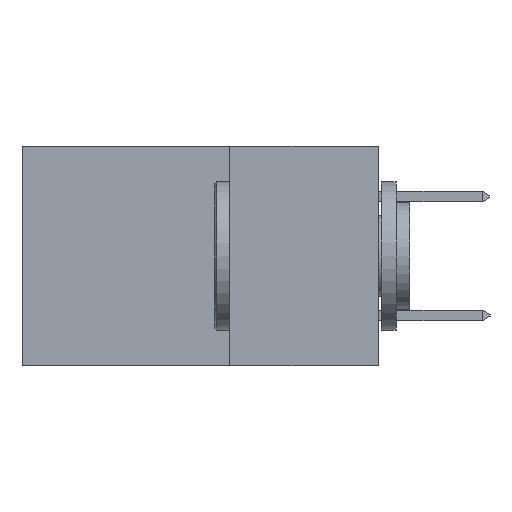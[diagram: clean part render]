
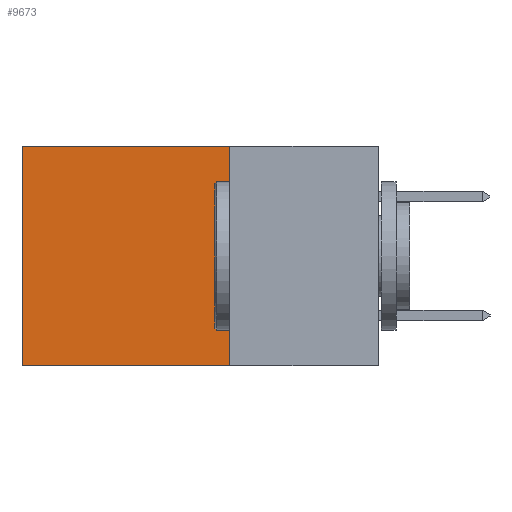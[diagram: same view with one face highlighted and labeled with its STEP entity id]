
A CAD part, left-side view. The second image highlights one B-rep face of the part: STEP entity #9673.
In plain terms, the highlighted planar face has unit normal (-1, 0, 0).
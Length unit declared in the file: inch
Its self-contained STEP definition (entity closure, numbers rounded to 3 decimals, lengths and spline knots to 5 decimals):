
#290 = DIRECTION ( 'NONE',  ( 0., 1., 0. ) ) ;
#348 = FACE_OUTER_BOUND ( 'NONE', #633, .T. ) ;
#394 = VECTOR ( 'NONE', #290, 39.37008 ) ;
#633 = EDGE_LOOP ( 'NONE', ( #13745, #1177, #6859, #8190 ) ) ;
#659 = CARTESIAN_POINT ( 'NONE',  ( 0.2615, 0.25, 0. ) ) ;
#821 = DIRECTION ( 'NONE',  ( 0., 0., -1. ) ) ;
#842 = LINE ( 'NONE', #9589, #10008 ) ;
#932 = CARTESIAN_POINT ( 'NONE',  ( 0.2615, 0.6, -0.37 ) ) ;
#1177 = ORIENTED_EDGE ( 'NONE', *, *, #11639, .F. ) ;
#1730 = AXIS2_PLACEMENT_3D ( 'NONE', #8292, #8228, #8213 ) ;
#2295 = CARTESIAN_POINT ( 'NONE',  ( 0.2615, 0.25, 0. ) ) ;
#2544 = VERTEX_POINT ( 'NONE', #4516 ) ;
#3401 = LINE ( 'NONE', #659, #394 ) ;
#4516 = CARTESIAN_POINT ( 'NONE',  ( 0.2615, 0.6, 0. ) ) ;
#4593 = EDGE_CURVE ( 'NONE', #2544, #13615, #6008, .T. ) ;
#4750 = LINE ( 'NONE', #6887, #7088 ) ;
#6008 = LINE ( 'NONE', #932, #13274 ) ;
#6738 = VERTEX_POINT ( 'NONE', #7807 ) ;
#6787 = DIRECTION ( 'NONE',  ( 0., 1., 0. ) ) ;
#6805 = CARTESIAN_POINT ( 'NONE',  ( 0.2615, 0.6, -0.37 ) ) ;
#6859 = ORIENTED_EDGE ( 'NONE', *, *, #8696, .F. ) ;
#6887 = CARTESIAN_POINT ( 'NONE',  ( 0.2615, 0.25, -0.37 ) ) ;
#7088 = VECTOR ( 'NONE', #6787, 39.37008 ) ;
#7589 = EDGE_CURVE ( 'NONE', #8982, #2544, #3401, .T. ) ;
#7807 = CARTESIAN_POINT ( 'NONE',  ( 0.2615, 0.25, -0.37 ) ) ;
#8190 = ORIENTED_EDGE ( 'NONE', *, *, #7589, .T. ) ;
#8213 = DIRECTION ( 'NONE',  ( 0., 0., -1. ) ) ;
#8228 = DIRECTION ( 'NONE',  ( 1., 0., 0. ) ) ;
#8292 = CARTESIAN_POINT ( 'NONE',  ( 0.2615, 0.25, -0.37 ) ) ;
#8379 = PLANE ( 'NONE',  #1730 ) ;
#8696 = EDGE_CURVE ( 'NONE', #8982, #6738, #842, .T. ) ;
#8982 = VERTEX_POINT ( 'NONE', #2295 ) ;
#9589 = CARTESIAN_POINT ( 'NONE',  ( 0.2615, 0.25, -0.37 ) ) ;
#9673 = ADVANCED_FACE ( 'NONE', ( #348 ), #8379, .F. ) ;
#9807 = DIRECTION ( 'NONE',  ( 0., 0., -1. ) ) ;
#10008 = VECTOR ( 'NONE', #9807, 39.37008 ) ;
#11639 = EDGE_CURVE ( 'NONE', #6738, #13615, #4750, .T. ) ;
#13274 = VECTOR ( 'NONE', #821, 39.37008 ) ;
#13615 = VERTEX_POINT ( 'NONE', #6805 ) ;
#13745 = ORIENTED_EDGE ( 'NONE', *, *, #4593, .T. ) ;
